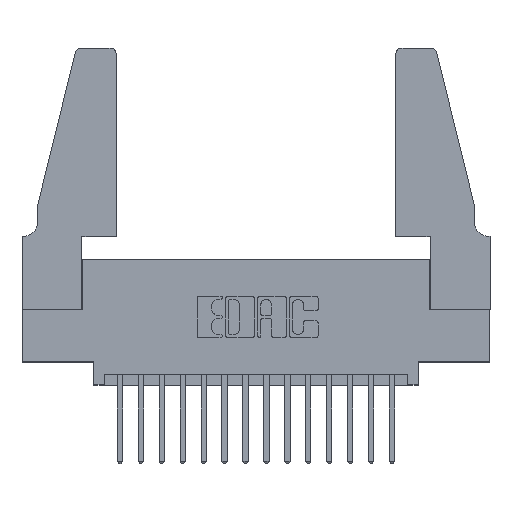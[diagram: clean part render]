
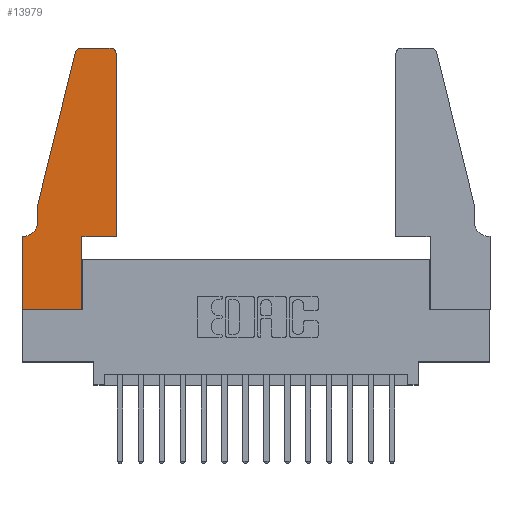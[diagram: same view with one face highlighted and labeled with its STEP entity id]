
A CAD part, top view. The second image highlights one B-rep face of the part: STEP entity #13979.
In plain terms, the highlighted planar face has unit normal (0, 0, 1).
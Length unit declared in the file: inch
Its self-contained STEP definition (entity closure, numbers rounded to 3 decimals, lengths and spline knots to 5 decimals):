
#23 = EDGE_CURVE ( 'NONE', #11765, #9581, #8379, .T. ) ;
#647 = DIRECTION ( 'NONE',  ( -1., 0., 0. ) ) ;
#705 = VECTOR ( 'NONE', #8679, 39.37008 ) ;
#1014 = CARTESIAN_POINT ( 'NONE',  ( 0.0755, 0.35, 0.37 ) ) ;
#1196 = DIRECTION ( 'NONE',  ( 1., 0., 0. ) ) ;
#1201 = DIRECTION ( 'NONE',  ( 0., -1., 0. ) ) ;
#1238 = VECTOR ( 'NONE', #15522, 39.37008 ) ;
#1367 = VECTOR ( 'NONE', #4943, 39.37008 ) ;
#1781 = VERTEX_POINT ( 'NONE', #4579 ) ;
#1966 = ORIENTED_EDGE ( 'NONE', *, *, #15067, .T. ) ;
#2000 = CIRCLE ( 'NONE', #9858, 0.03 ) ;
#2247 = CIRCLE ( 'NONE', #3493, 0.07 ) ;
#2515 = AXIS2_PLACEMENT_3D ( 'NONE', #16909, #9265, #1196 ) ;
#2592 = EDGE_CURVE ( 'NONE', #16328, #1781, #15577, .T. ) ;
#2818 = CARTESIAN_POINT ( 'NONE',  ( 0.0055, 0.42, 0.37 ) ) ;
#3060 = DIRECTION ( 'NONE',  ( 0., 0., 1. ) ) ;
#3103 = EDGE_CURVE ( 'NONE', #9969, #11765, #7873, .T. ) ;
#3409 = EDGE_CURVE ( 'NONE', #16714, #16851, #10374, .T. ) ;
#3493 = AXIS2_PLACEMENT_3D ( 'NONE', #2818, #12138, #4175 ) ;
#4175 = DIRECTION ( 'NONE',  ( -1., 0., 0. ) ) ;
#4579 = CARTESIAN_POINT ( 'NONE',  ( 0.4505, 0.35, 0.37 ) ) ;
#4943 = DIRECTION ( 'NONE',  ( 0., 1., 0. ) ) ;
#5356 = CARTESIAN_POINT ( 'NONE',  ( 0.284, 1.22, 0.37 ) ) ;
#5600 = ORIENTED_EDGE ( 'NONE', *, *, #13151, .T. ) ;
#5759 = LINE ( 'NONE', #16407, #15694 ) ;
#6032 = CARTESIAN_POINT ( 'NONE',  ( 0., 0., 0.37 ) ) ;
#6038 = VERTEX_POINT ( 'NONE', #9342 ) ;
#6126 = EDGE_CURVE ( 'NONE', #16369, #14567, #2247, .T. ) ;
#6267 = CARTESIAN_POINT ( 'NONE',  ( 0., 0., 0.37 ) ) ;
#6611 = CARTESIAN_POINT ( 'NONE',  ( 0.284, 1.25, 0.37 ) ) ;
#6679 = DIRECTION ( 'NONE',  ( 1., 0., 0. ) ) ;
#6841 = ORIENTED_EDGE ( 'NONE', *, *, #23, .T. ) ;
#6935 = CARTESIAN_POINT ( 'NONE',  ( 0., 0., 0.37 ) ) ;
#6967 = EDGE_CURVE ( 'NONE', #1781, #16714, #16567, .T. ) ;
#7873 = LINE ( 'NONE', #6032, #705 ) ;
#7887 = VECTOR ( 'NONE', #16669, 39.37008 ) ;
#8040 = VERTEX_POINT ( 'NONE', #14843 ) ;
#8322 = PLANE ( 'NONE',  #14082 ) ;
#8379 = LINE ( 'NONE', #6935, #11484 ) ;
#8483 = DIRECTION ( 'NONE',  ( 1., 0., 0. ) ) ;
#8679 = DIRECTION ( 'NONE',  ( 0., -1., 0. ) ) ;
#8854 = CARTESIAN_POINT ( 'NONE',  ( 0.2865, 0., 0.37 ) ) ;
#9079 = DIRECTION ( 'NONE',  ( -1., 0., 0. ) ) ;
#9090 = VERTEX_POINT ( 'NONE', #6611 ) ;
#9125 = ORIENTED_EDGE ( 'NONE', *, *, #10242, .T. ) ;
#9244 = VECTOR ( 'NONE', #9079, 39.37008 ) ;
#9265 = DIRECTION ( 'NONE',  ( 0., 0., 1. ) ) ;
#9342 = CARTESIAN_POINT ( 'NONE',  ( 0.25487, 1.22718, 0.37 ) ) ;
#9372 = LINE ( 'NONE', #11543, #1367 ) ;
#9541 = ORIENTED_EDGE ( 'NONE', *, *, #14659, .T. ) ;
#9581 = VERTEX_POINT ( 'NONE', #8854 ) ;
#9833 = CARTESIAN_POINT ( 'NONE',  ( 0., 0.35, 0.37 ) ) ;
#9858 = AXIS2_PLACEMENT_3D ( 'NONE', #5356, #14479, #6679 ) ;
#9954 = ORIENTED_EDGE ( 'NONE', *, *, #17011, .T. ) ;
#9969 = VERTEX_POINT ( 'NONE', #9833 ) ;
#10076 = LINE ( 'NONE', #1014, #9244 ) ;
#10178 = DIRECTION ( 'NONE',  ( 0., 1., 0. ) ) ;
#10242 = EDGE_CURVE ( 'NONE', #6038, #8040, #16057, .T. ) ;
#10371 = ORIENTED_EDGE ( 'NONE', *, *, #12934, .T. ) ;
#10372 = CARTESIAN_POINT ( 'NONE',  ( 0.0055, 0.35, 0.37 ) ) ;
#10374 = CIRCLE ( 'NONE', #2515, 0.03 ) ;
#10791 = ORIENTED_EDGE ( 'NONE', *, *, #6967, .T. ) ;
#11484 = VECTOR ( 'NONE', #8483, 39.37008 ) ;
#11543 = CARTESIAN_POINT ( 'NONE',  ( 0.2865, 0.35, 0.37 ) ) ;
#11628 = CARTESIAN_POINT ( 'NONE',  ( 0.0755, 0.42, 0.37 ) ) ;
#11765 = VERTEX_POINT ( 'NONE', #6267 ) ;
#11967 = VECTOR ( 'NONE', #1201, 39.37008 ) ;
#12138 = DIRECTION ( 'NONE',  ( 0., 0., -1. ) ) ;
#12348 = CARTESIAN_POINT ( 'NONE',  ( 0.4505, 1.22, 0.37 ) ) ;
#12352 = DIRECTION ( 'NONE',  ( 1., 0., 0. ) ) ;
#12869 = CARTESIAN_POINT ( 'NONE',  ( 0.4505, 0.35, 0.37 ) ) ;
#12934 = EDGE_CURVE ( 'NONE', #9581, #16328, #9372, .T. ) ;
#12987 = ORIENTED_EDGE ( 'NONE', *, *, #6126, .T. ) ;
#13151 = EDGE_CURVE ( 'NONE', #9090, #6038, #2000, .T. ) ;
#13216 = VECTOR ( 'NONE', #10178, 39.37008 ) ;
#13381 = ORIENTED_EDGE ( 'NONE', *, *, #3103, .T. ) ;
#13789 = ORIENTED_EDGE ( 'NONE', *, *, #2592, .T. ) ;
#13888 = CARTESIAN_POINT ( 'NONE',  ( 0.4205, 1.25, 0.37 ) ) ;
#13979 = ADVANCED_FACE ( 'NONE', ( #16327 ), #8322, .T. ) ;
#14082 = AXIS2_PLACEMENT_3D ( 'NONE', #14832, #3060, #12352 ) ;
#14188 = ORIENTED_EDGE ( 'NONE', *, *, #3409, .T. ) ;
#14271 = CARTESIAN_POINT ( 'NONE',  ( 0.0755, 0.5, 0.37 ) ) ;
#14479 = DIRECTION ( 'NONE',  ( 0., 0., 1. ) ) ;
#14567 = VERTEX_POINT ( 'NONE', #10372 ) ;
#14659 = EDGE_CURVE ( 'NONE', #8040, #16369, #15715, .T. ) ;
#14832 = CARTESIAN_POINT ( 'NONE',  ( 0., 0.35, 0.37 ) ) ;
#14843 = CARTESIAN_POINT ( 'NONE',  ( 0.0755, 0.5, 0.37 ) ) ;
#15067 = EDGE_CURVE ( 'NONE', #16851, #9090, #5759, .T. ) ;
#15336 = CARTESIAN_POINT ( 'NONE',  ( 0.2865, 0.35, 0.37 ) ) ;
#15452 = EDGE_LOOP ( 'NONE', ( #1966, #5600, #9125, #9541, #12987, #9954, #13381, #6841, #10371, #13789, #10791, #14188 ) ) ;
#15522 = DIRECTION ( 'NONE',  ( -0.239, -0.971, 0. ) ) ;
#15577 = LINE ( 'NONE', #12869, #7887 ) ;
#15694 = VECTOR ( 'NONE', #647, 39.37008 ) ;
#15715 = LINE ( 'NONE', #16915, #11967 ) ;
#16057 = LINE ( 'NONE', #14271, #1238 ) ;
#16327 = FACE_OUTER_BOUND ( 'NONE', #15452, .T. ) ;
#16328 = VERTEX_POINT ( 'NONE', #15336 ) ;
#16369 = VERTEX_POINT ( 'NONE', #11628 ) ;
#16407 = CARTESIAN_POINT ( 'NONE',  ( 0.2605, 1.25, 0.37 ) ) ;
#16524 = CARTESIAN_POINT ( 'NONE',  ( 0.4505, 0.35, 0.37 ) ) ;
#16567 = LINE ( 'NONE', #16524, #13216 ) ;
#16669 = DIRECTION ( 'NONE',  ( 1., 0., 0. ) ) ;
#16714 = VERTEX_POINT ( 'NONE', #12348 ) ;
#16851 = VERTEX_POINT ( 'NONE', #13888 ) ;
#16909 = CARTESIAN_POINT ( 'NONE',  ( 0.4205, 1.22, 0.37 ) ) ;
#16915 = CARTESIAN_POINT ( 'NONE',  ( 0.0755, 0.5, 0.37 ) ) ;
#17011 = EDGE_CURVE ( 'NONE', #14567, #9969, #10076, .T. ) ;
